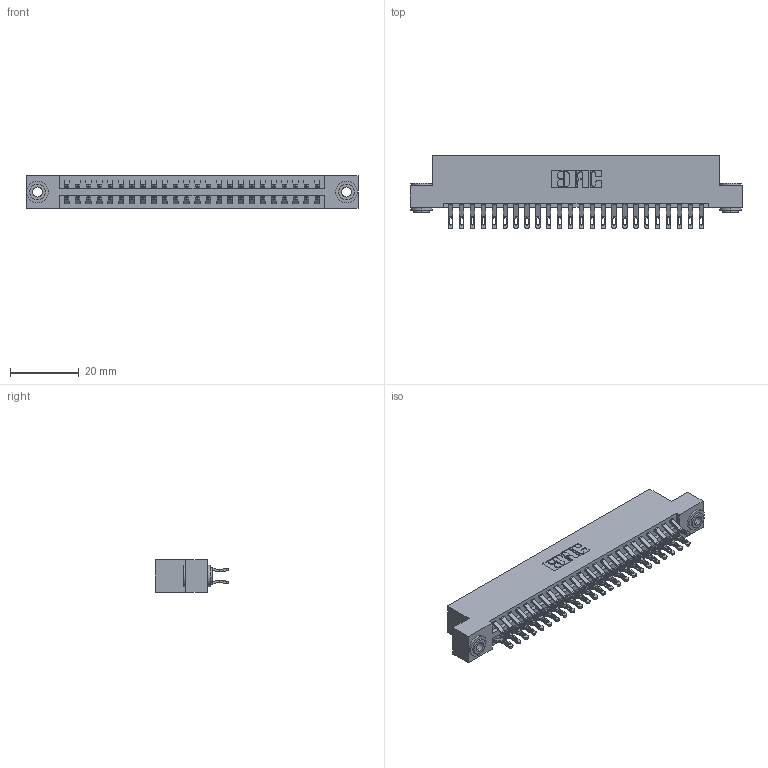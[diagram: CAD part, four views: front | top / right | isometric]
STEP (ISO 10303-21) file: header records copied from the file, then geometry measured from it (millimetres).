
FILE_DESCRIPTION (( 'STEP AP203' ), '1' );
FILE_NAME ('346-048-555-203.STEP', '2018-08-25T10:25:35', ( '' ), ( '' ), 'SwSTEP 2.0', 'SolidWorks 2016', '' );
FILE_SCHEMA (( 'CONFIG_CONTROL_DESIGN' ));
Length unit declared in the file: inch
Products named in the file (4): 345-292-001_555 Tail; 345-250-002_345-250-002-102; 346-048-555-203; 346 Part_Flush Mounting Lugs - 0.156 Dia-TH
Assembly tree (51 placements, depth 2):
  346-048-555-203
    346 Part_Flush Mounting Lugs - 0.156 Dia-TH
    345-292-001_555 Tail  x48
    345-250-002_345-250-002-102  x2
Bounding box: 96.77 x 21.46 x 9.4 mm (x, y, z)
Volume: 9455.5 mm3; surface area: 13424.8 mm2
Topology: 51 solids, 51 shells, 2944 faces, 9189 edges, 6122 vertices
Faces by surface type: plane 1670, cylinder 1266, cone 8
Entity records: 19062 total; most frequent: CARTESIAN_POINT 3177, ORIENTED_EDGE 3074, DIRECTION 2851, EDGE_CURVE 1537, VECTOR 1265, LINE 1265, VERTEX_POINT 1022, AXIS2_PLACEMENT_3D 793
